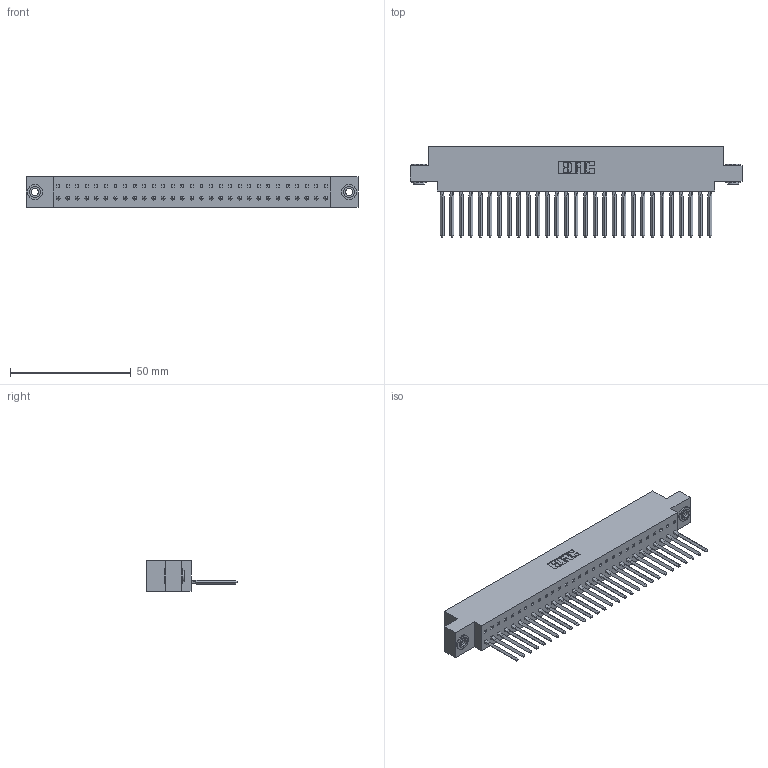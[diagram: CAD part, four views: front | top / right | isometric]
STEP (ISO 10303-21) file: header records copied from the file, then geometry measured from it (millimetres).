
FILE_DESCRIPTION (( 'STEP AP203' ), '1' );
FILE_NAME ('317-029-541-603.STEP', '2020-02-27T19:59:34', ( '' ), ( '' ), 'SwSTEP 2.0', 'SolidWorks 2016', '' );
FILE_SCHEMA (( 'CONFIG_CONTROL_DESIGN' ));
Length unit declared in the file: inch
Products named in the file (4): 317-029-541-603; 345-250-002_345-250-002-102; 317 Part_.156 Dia - TH; 317-290-002_541
Assembly tree (32 placements, depth 2):
  317-029-541-603
    317 Part_.156 Dia - TH
    317-290-002_541  x29
    345-250-002_345-250-002-102  x2
Bounding box: 137.62 x 37.34 x 12.7 mm (x, y, z)
Volume: 21936.6 mm3; surface area: 30779.1 mm2
Topology: 32 solids, 32 shells, 4548 faces, 12937 edges, 8408 vertices
Faces by surface type: plane 3664, cylinder 760, bspline 116, cone 8
Entity records: 45003 total; most frequent: CARTESIAN_POINT 8603, ORIENTED_EDGE 7878, DIRECTION 6503, EDGE_CURVE 3939, LINE 3551, VECTOR 3551, VERTEX_POINT 2616, AXIS2_PLACEMENT_3D 1476
